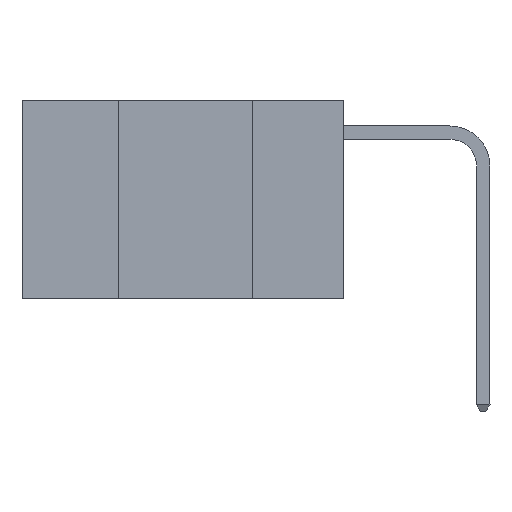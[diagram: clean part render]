
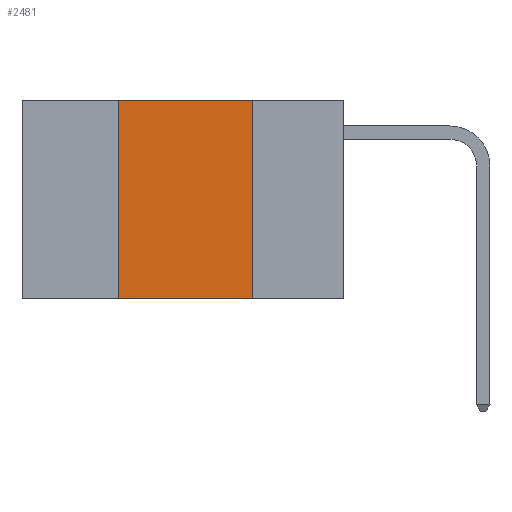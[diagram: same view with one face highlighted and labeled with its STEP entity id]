
A CAD part, left-side view. The second image highlights one B-rep face of the part: STEP entity #2481.
In plain terms, the highlighted planar face has unit normal (-1, 0, 0).
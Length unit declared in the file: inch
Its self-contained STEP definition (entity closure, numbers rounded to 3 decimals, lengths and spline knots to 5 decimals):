
#211 = CARTESIAN_POINT ( 'NONE',  ( 0., 0.42, 0. ) ) ;
#385 = EDGE_CURVE ( 'NONE', #458, #6956, #14009, .T. ) ;
#458 = VERTEX_POINT ( 'NONE', #11701 ) ;
#656 = DIRECTION ( 'NONE',  ( 0., 0., -1. ) ) ;
#1597 = LINE ( 'NONE', #13521, #10168 ) ;
#2002 = CARTESIAN_POINT ( 'NONE',  ( 0., 0.6, 0. ) ) ;
#2481 = ADVANCED_FACE ( 'NONE', ( #6168 ), #11702, .F. ) ;
#2771 = DIRECTION ( 'NONE',  ( 0., -1., 0. ) ) ;
#2834 = EDGE_CURVE ( 'NONE', #6332, #9349, #6045, .T. ) ;
#2904 = CARTESIAN_POINT ( 'NONE',  ( 0., 0.17, -0.37 ) ) ;
#3680 = VECTOR ( 'NONE', #12247, 39.37008 ) ;
#3821 = DIRECTION ( 'NONE',  ( 0., -1., 0. ) ) ;
#3892 = CARTESIAN_POINT ( 'NONE',  ( 0., 0.42, 0. ) ) ;
#4680 = EDGE_LOOP ( 'NONE', ( #13329, #4941, #9088, #12068 ) ) ;
#4851 = AXIS2_PLACEMENT_3D ( 'NONE', #2002, #12894, #9639 ) ;
#4941 = ORIENTED_EDGE ( 'NONE', *, *, #6117, .F. ) ;
#5028 = CARTESIAN_POINT ( 'NONE',  ( 0., 0.6, -0.37 ) ) ;
#5238 = VECTOR ( 'NONE', #3821, 39.37008 ) ;
#5738 = VECTOR ( 'NONE', #656, 39.37008 ) ;
#6045 = LINE ( 'NONE', #12772, #5738 ) ;
#6117 = EDGE_CURVE ( 'NONE', #6956, #6332, #1597, .T. ) ;
#6168 = FACE_OUTER_BOUND ( 'NONE', #4680, .T. ) ;
#6332 = VERTEX_POINT ( 'NONE', #13918 ) ;
#6956 = VERTEX_POINT ( 'NONE', #3892 ) ;
#9088 = ORIENTED_EDGE ( 'NONE', *, *, #385, .F. ) ;
#9349 = VERTEX_POINT ( 'NONE', #2904 ) ;
#9639 = DIRECTION ( 'NONE',  ( 0., 0., -1. ) ) ;
#10168 = VECTOR ( 'NONE', #2771, 39.37008 ) ;
#11466 = LINE ( 'NONE', #5028, #5238 ) ;
#11701 = CARTESIAN_POINT ( 'NONE',  ( 0., 0.42, -0.37 ) ) ;
#11702 = PLANE ( 'NONE',  #4851 ) ;
#12068 = ORIENTED_EDGE ( 'NONE', *, *, #13694, .T. ) ;
#12247 = DIRECTION ( 'NONE',  ( 0., 0., 1. ) ) ;
#12772 = CARTESIAN_POINT ( 'NONE',  ( 0., 0.17, 0. ) ) ;
#12894 = DIRECTION ( 'NONE',  ( 1., 0., 0. ) ) ;
#13329 = ORIENTED_EDGE ( 'NONE', *, *, #2834, .F. ) ;
#13521 = CARTESIAN_POINT ( 'NONE',  ( 0., 0.6, 0. ) ) ;
#13694 = EDGE_CURVE ( 'NONE', #458, #9349, #11466, .T. ) ;
#13918 = CARTESIAN_POINT ( 'NONE',  ( 0., 0.17, 0. ) ) ;
#14009 = LINE ( 'NONE', #211, #3680 ) ;
